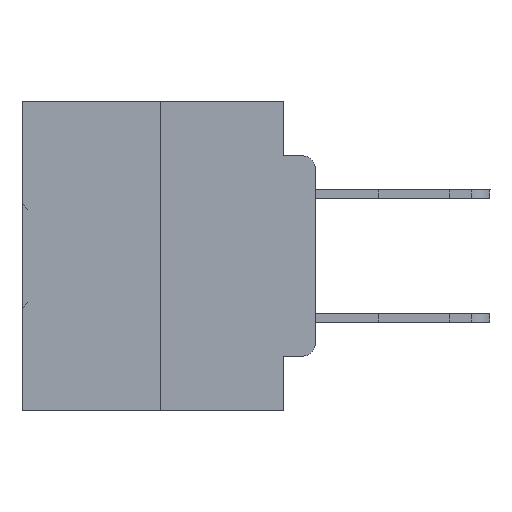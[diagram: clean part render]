
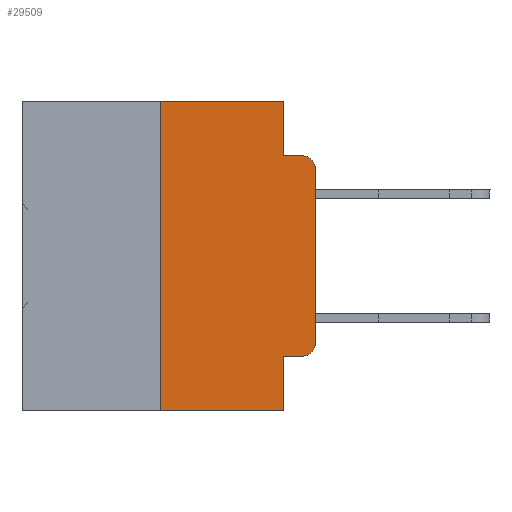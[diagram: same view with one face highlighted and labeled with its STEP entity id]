
A CAD part, left-side view. The second image highlights one B-rep face of the part: STEP entity #29509.
In plain terms, the highlighted planar face has unit normal (-1, 0, 0).
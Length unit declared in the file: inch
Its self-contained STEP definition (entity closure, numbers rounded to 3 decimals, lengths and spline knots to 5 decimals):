
#28 = DIRECTION ( 'NONE',  ( 0., 0., -1. ) ) ;
#87 = LINE ( 'NONE', #33488, #30518 ) ;
#194 = DIRECTION ( 'NONE',  ( 0., 0., -1. ) ) ;
#499 = ORIENTED_EDGE ( 'NONE', *, *, #14285, .T. ) ;
#797 = LINE ( 'NONE', #8473, #1260 ) ;
#1260 = VECTOR ( 'NONE', #194, 39.37008 ) ;
#3593 = VERTEX_POINT ( 'NONE', #10990 ) ;
#3665 = EDGE_CURVE ( 'NONE', #36554, #34718, #797, .T. ) ;
#3745 = CIRCLE ( 'NONE', #34667, 0.02 ) ;
#3850 = EDGE_CURVE ( 'NONE', #3593, #33970, #33897, .T. ) ;
#4165 = EDGE_CURVE ( 'NONE', #34718, #30798, #34745, .T. ) ;
#4388 = DIRECTION ( 'NONE',  ( 0., -1., 0. ) ) ;
#4435 = ORIENTED_EDGE ( 'NONE', *, *, #4165, .F. ) ;
#4524 = CARTESIAN_POINT ( 'NONE',  ( 0., 0.051, -0.0885 ) ) ;
#4929 = EDGE_CURVE ( 'NONE', #16586, #11641, #27170, .T. ) ;
#5202 = DIRECTION ( 'NONE',  ( 0., 0., -1. ) ) ;
#5411 = FACE_OUTER_BOUND ( 'NONE', #11485, .T. ) ;
#5694 = CARTESIAN_POINT ( 'NONE',  ( 0., 0.02, -0.3915 ) ) ;
#7549 = ORIENTED_EDGE ( 'NONE', *, *, #11656, .T. ) ;
#7846 = CARTESIAN_POINT ( 'NONE',  ( 0., 0.02, -0.1085 ) ) ;
#7913 = ORIENTED_EDGE ( 'NONE', *, *, #3665, .F. ) ;
#8269 = VECTOR ( 'NONE', #4388, 39.37008 ) ;
#8473 = CARTESIAN_POINT ( 'NONE',  ( 0., 0.051, 0. ) ) ;
#8721 = DIRECTION ( 'NONE',  ( 0., 0., 1. ) ) ;
#9938 = CARTESIAN_POINT ( 'NONE',  ( 0., 0., -0.1085 ) ) ;
#10074 = CARTESIAN_POINT ( 'NONE',  ( 0., 0.051, -0.0885 ) ) ;
#10341 = EDGE_CURVE ( 'NONE', #16946, #24486, #22066, .T. ) ;
#10476 = LINE ( 'NONE', #25148, #26338 ) ;
#10788 = DIRECTION ( 'NONE',  ( -1., 0., 0. ) ) ;
#10990 = CARTESIAN_POINT ( 'NONE',  ( 0., 0.25, -0.5 ) ) ;
#11356 = EDGE_CURVE ( 'NONE', #33970, #36554, #33137, .T. ) ;
#11481 = CARTESIAN_POINT ( 'NONE',  ( 0., 0.02, -0.0885 ) ) ;
#11485 = EDGE_LOOP ( 'NONE', ( #32605, #7549, #4435, #7913, #21228, #35405, #28228, #13697, #11947, #499 ) ) ;
#11641 = VERTEX_POINT ( 'NONE', #9938 ) ;
#11656 = EDGE_CURVE ( 'NONE', #11641, #30798, #30416, .T. ) ;
#11685 = CARTESIAN_POINT ( 'NONE',  ( 0., 0., 0. ) ) ;
#11937 = CARTESIAN_POINT ( 'NONE',  ( 0., 0.25, 0. ) ) ;
#11947 = ORIENTED_EDGE ( 'NONE', *, *, #29994, .T. ) ;
#12596 = CARTESIAN_POINT ( 'NONE',  ( 0., 0.25, 0. ) ) ;
#12700 = VECTOR ( 'NONE', #31520, 39.37008 ) ;
#13697 = ORIENTED_EDGE ( 'NONE', *, *, #10341, .F. ) ;
#13714 = VECTOR ( 'NONE', #28, 39.37008 ) ;
#14285 = EDGE_CURVE ( 'NONE', #15738, #16586, #3745, .T. ) ;
#15738 = VERTEX_POINT ( 'NONE', #29757 ) ;
#16586 = VERTEX_POINT ( 'NONE', #22507 ) ;
#16946 = VERTEX_POINT ( 'NONE', #24344 ) ;
#17271 = CARTESIAN_POINT ( 'NONE',  ( 0., 0.473, 0. ) ) ;
#20901 = DIRECTION ( 'NONE',  ( 0., -1., 0. ) ) ;
#21228 = ORIENTED_EDGE ( 'NONE', *, *, #11356, .F. ) ;
#21733 = CARTESIAN_POINT ( 'NONE',  ( 0., 0.051, 0. ) ) ;
#21856 = VECTOR ( 'NONE', #8721, 39.37008 ) ;
#22066 = LINE ( 'NONE', #36320, #13714 ) ;
#22507 = CARTESIAN_POINT ( 'NONE',  ( 0., 0., -0.3915 ) ) ;
#22896 = VECTOR ( 'NONE', #20901, 39.37008 ) ;
#23052 = DIRECTION ( 'NONE',  ( 0., 0., -1. ) ) ;
#24344 = CARTESIAN_POINT ( 'NONE',  ( 0., 0.051, -0.4115 ) ) ;
#24486 = VERTEX_POINT ( 'NONE', #27885 ) ;
#24946 = AXIS2_PLACEMENT_3D ( 'NONE', #17271, #25803, #23052 ) ;
#25148 = CARTESIAN_POINT ( 'NONE',  ( 0., 0.473, -0.5 ) ) ;
#25803 = DIRECTION ( 'NONE',  ( 1., 0., 0. ) ) ;
#26338 = VECTOR ( 'NONE', #33693, 39.37008 ) ;
#26722 = CARTESIAN_POINT ( 'NONE',  ( 0., 0.473, 0. ) ) ;
#27170 = LINE ( 'NONE', #11685, #21856 ) ;
#27885 = CARTESIAN_POINT ( 'NONE',  ( 0., 0.051, -0.5 ) ) ;
#28228 = ORIENTED_EDGE ( 'NONE', *, *, #32530, .T. ) ;
#29509 = ADVANCED_FACE ( 'NONE', ( #5411 ), #34350, .F. ) ;
#29757 = CARTESIAN_POINT ( 'NONE',  ( 0., 0.02, -0.4115 ) ) ;
#29994 = EDGE_CURVE ( 'NONE', #16946, #15738, #87, .T. ) ;
#30416 = CIRCLE ( 'NONE', #33472, 0.02 ) ;
#30518 = VECTOR ( 'NONE', #32797, 39.37008 ) ;
#30798 = VERTEX_POINT ( 'NONE', #11481 ) ;
#31520 = DIRECTION ( 'NONE',  ( 0., 0., 1. ) ) ;
#32530 = EDGE_CURVE ( 'NONE', #3593, #24486, #10476, .T. ) ;
#32605 = ORIENTED_EDGE ( 'NONE', *, *, #4929, .T. ) ;
#32797 = DIRECTION ( 'NONE',  ( 0., -1., 0. ) ) ;
#32885 = DIRECTION ( 'NONE',  ( 0., 0., -1. ) ) ;
#33137 = LINE ( 'NONE', #26722, #22896 ) ;
#33472 = AXIS2_PLACEMENT_3D ( 'NONE', #7846, #10788, #32885 ) ;
#33488 = CARTESIAN_POINT ( 'NONE',  ( 0., 0.051, -0.4115 ) ) ;
#33693 = DIRECTION ( 'NONE',  ( 0., -1., 0. ) ) ;
#33897 = LINE ( 'NONE', #11937, #12700 ) ;
#33970 = VERTEX_POINT ( 'NONE', #12596 ) ;
#34350 = PLANE ( 'NONE',  #24946 ) ;
#34667 = AXIS2_PLACEMENT_3D ( 'NONE', #5694, #36295, #5202 ) ;
#34718 = VERTEX_POINT ( 'NONE', #10074 ) ;
#34745 = LINE ( 'NONE', #4524, #8269 ) ;
#35405 = ORIENTED_EDGE ( 'NONE', *, *, #3850, .F. ) ;
#36295 = DIRECTION ( 'NONE',  ( -1., 0., 0. ) ) ;
#36320 = CARTESIAN_POINT ( 'NONE',  ( 0., 0.051, 0. ) ) ;
#36554 = VERTEX_POINT ( 'NONE', #21733 ) ;
